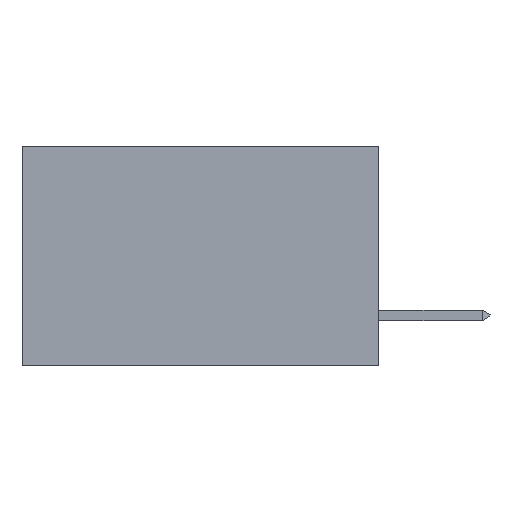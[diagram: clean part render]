
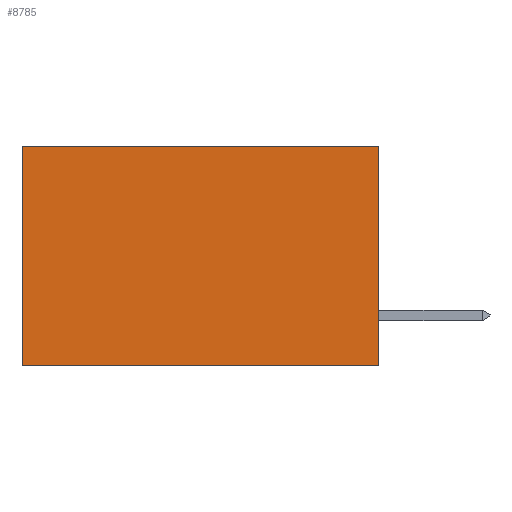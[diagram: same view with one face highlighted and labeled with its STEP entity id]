
A CAD part, left-side view. The second image highlights one B-rep face of the part: STEP entity #8785.
In plain terms, the highlighted planar face has unit normal (-1, 0, 0).
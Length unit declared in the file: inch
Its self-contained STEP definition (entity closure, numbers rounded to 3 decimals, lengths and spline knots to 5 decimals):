
#244 = ORIENTED_EDGE ( 'NONE', *, *, #6025, .F. ) ;
#370 = CARTESIAN_POINT ( 'NONE',  ( 0.2615, 0., 0. ) ) ;
#693 = CARTESIAN_POINT ( 'NONE',  ( 0.2615, 0.6, -0.37 ) ) ;
#905 = LINE ( 'NONE', #9030, #10269 ) ;
#977 = DIRECTION ( 'NONE',  ( 0., 0., -1. ) ) ;
#1112 = ORIENTED_EDGE ( 'NONE', *, *, #2594, .T. ) ;
#1235 = EDGE_LOOP ( 'NONE', ( #1112, #244, #2466, #1360 ) ) ;
#1360 = ORIENTED_EDGE ( 'NONE', *, *, #1374, .T. ) ;
#1374 = EDGE_CURVE ( 'NONE', #6070, #1537, #7172, .T. ) ;
#1537 = VERTEX_POINT ( 'NONE', #9497 ) ;
#1648 = VERTEX_POINT ( 'NONE', #11358 ) ;
#1925 = CARTESIAN_POINT ( 'NONE',  ( 0.2615, 0., 0. ) ) ;
#2324 = PLANE ( 'NONE',  #9579 ) ;
#2466 = ORIENTED_EDGE ( 'NONE', *, *, #8951, .F. ) ;
#2497 = VERTEX_POINT ( 'NONE', #693 ) ;
#2594 = EDGE_CURVE ( 'NONE', #1537, #2497, #5559, .T. ) ;
#2889 = CARTESIAN_POINT ( 'NONE',  ( 0.2615, 0.6, -0.37 ) ) ;
#3631 = DIRECTION ( 'NONE',  ( 0., 1., 0. ) ) ;
#5021 = CARTESIAN_POINT ( 'NONE',  ( 0.2615, 0., -0.37 ) ) ;
#5544 = VECTOR ( 'NONE', #977, 39.37008 ) ;
#5559 = LINE ( 'NONE', #2889, #5544 ) ;
#6025 = EDGE_CURVE ( 'NONE', #1648, #2497, #905, .T. ) ;
#6070 = VERTEX_POINT ( 'NONE', #1925 ) ;
#7172 = LINE ( 'NONE', #370, #7507 ) ;
#7507 = VECTOR ( 'NONE', #3631, 39.37008 ) ;
#7889 = VECTOR ( 'NONE', #11515, 39.37008 ) ;
#8785 = ADVANCED_FACE ( 'NONE', ( #10368 ), #2324, .F. ) ;
#8829 = LINE ( 'NONE', #11398, #7889 ) ;
#8857 = DIRECTION ( 'NONE',  ( 0., 1., 0. ) ) ;
#8951 = EDGE_CURVE ( 'NONE', #6070, #1648, #8829, .T. ) ;
#9030 = CARTESIAN_POINT ( 'NONE',  ( 0.2615, 0., -0.37 ) ) ;
#9489 = DIRECTION ( 'NONE',  ( 1., 0., 0. ) ) ;
#9497 = CARTESIAN_POINT ( 'NONE',  ( 0.2615, 0.6, 0. ) ) ;
#9579 = AXIS2_PLACEMENT_3D ( 'NONE', #5021, #9489, #11186 ) ;
#10269 = VECTOR ( 'NONE', #8857, 39.37008 ) ;
#10368 = FACE_OUTER_BOUND ( 'NONE', #1235, .T. ) ;
#11186 = DIRECTION ( 'NONE',  ( 0., 0., -1. ) ) ;
#11358 = CARTESIAN_POINT ( 'NONE',  ( 0.2615, 0., -0.37 ) ) ;
#11398 = CARTESIAN_POINT ( 'NONE',  ( 0.2615, 0., -0.37 ) ) ;
#11515 = DIRECTION ( 'NONE',  ( 0., 0., -1. ) ) ;
